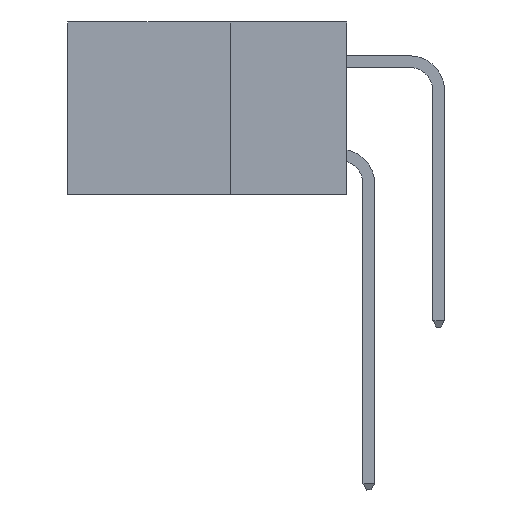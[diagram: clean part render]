
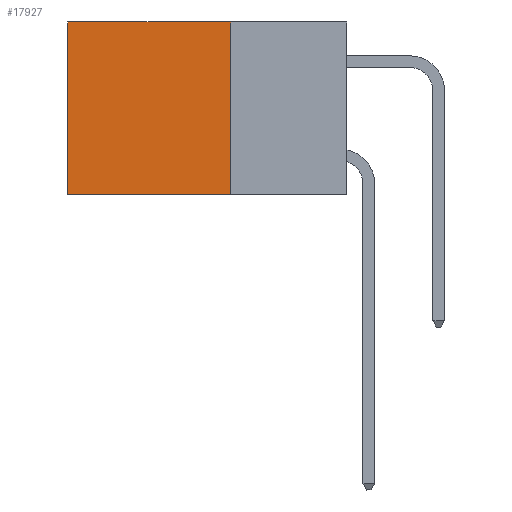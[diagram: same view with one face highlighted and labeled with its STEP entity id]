
A CAD part, left-side view. The second image highlights one B-rep face of the part: STEP entity #17927.
In plain terms, the highlighted planar face has unit normal (-1, 0, 0).
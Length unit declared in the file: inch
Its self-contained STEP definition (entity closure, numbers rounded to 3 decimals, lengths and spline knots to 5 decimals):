
#839 = AXIS2_PLACEMENT_3D ( 'NONE', #17073, #7170, #18663 ) ;
#1329 = VERTEX_POINT ( 'NONE', #5710 ) ;
#2319 = CARTESIAN_POINT ( 'NONE',  ( 0.2875, 0.25, 0. ) ) ;
#2384 = EDGE_LOOP ( 'NONE', ( #11455, #5122, #5774, #20100 ) ) ;
#2768 = EDGE_CURVE ( 'NONE', #6726, #14631, #6128, .T. ) ;
#2894 = EDGE_CURVE ( 'NONE', #6726, #21035, #7443, .T. ) ;
#2928 = VECTOR ( 'NONE', #13350, 39.37008 ) ;
#4074 = VECTOR ( 'NONE', #8537, 39.37008 ) ;
#4603 = CARTESIAN_POINT ( 'NONE',  ( 0.2875, 0.25, -0.37 ) ) ;
#5122 = ORIENTED_EDGE ( 'NONE', *, *, #6251, .F. ) ;
#5710 = CARTESIAN_POINT ( 'NONE',  ( 0.2875, 0.6, -0.37 ) ) ;
#5774 = ORIENTED_EDGE ( 'NONE', *, *, #2894, .F. ) ;
#6128 = LINE ( 'NONE', #17945, #14003 ) ;
#6251 = EDGE_CURVE ( 'NONE', #21035, #1329, #7562, .T. ) ;
#6288 = DIRECTION ( 'NONE',  ( 0., 1., 0. ) ) ;
#6726 = VERTEX_POINT ( 'NONE', #2319 ) ;
#7116 = EDGE_CURVE ( 'NONE', #14631, #1329, #17323, .T. ) ;
#7170 = DIRECTION ( 'NONE',  ( 1., 0., 0. ) ) ;
#7443 = LINE ( 'NONE', #11685, #2928 ) ;
#7562 = LINE ( 'NONE', #4603, #15851 ) ;
#8002 = CARTESIAN_POINT ( 'NONE',  ( 0.2875, 0.6, 0. ) ) ;
#8537 = DIRECTION ( 'NONE',  ( 0., 0., -1. ) ) ;
#8856 = PLANE ( 'NONE',  #839 ) ;
#11455 = ORIENTED_EDGE ( 'NONE', *, *, #7116, .T. ) ;
#11685 = CARTESIAN_POINT ( 'NONE',  ( 0.2875, 0.25, 0. ) ) ;
#12640 = FACE_OUTER_BOUND ( 'NONE', #2384, .T. ) ;
#13074 = DIRECTION ( 'NONE',  ( 0., 1., 0. ) ) ;
#13350 = DIRECTION ( 'NONE',  ( 0., 0., -1. ) ) ;
#14003 = VECTOR ( 'NONE', #13074, 39.37008 ) ;
#14631 = VERTEX_POINT ( 'NONE', #8002 ) ;
#15851 = VECTOR ( 'NONE', #6288, 39.37008 ) ;
#17073 = CARTESIAN_POINT ( 'NONE',  ( 0.2875, 0.25, 0. ) ) ;
#17323 = LINE ( 'NONE', #18309, #4074 ) ;
#17927 = ADVANCED_FACE ( 'NONE', ( #12640 ), #8856, .F. ) ;
#17945 = CARTESIAN_POINT ( 'NONE',  ( 0.2875, 0.25, 0. ) ) ;
#18309 = CARTESIAN_POINT ( 'NONE',  ( 0.2875, 0.6, 0. ) ) ;
#18663 = DIRECTION ( 'NONE',  ( 0., 0., -1. ) ) ;
#20100 = ORIENTED_EDGE ( 'NONE', *, *, #2768, .T. ) ;
#21035 = VERTEX_POINT ( 'NONE', #21074 ) ;
#21074 = CARTESIAN_POINT ( 'NONE',  ( 0.2875, 0.25, -0.37 ) ) ;
